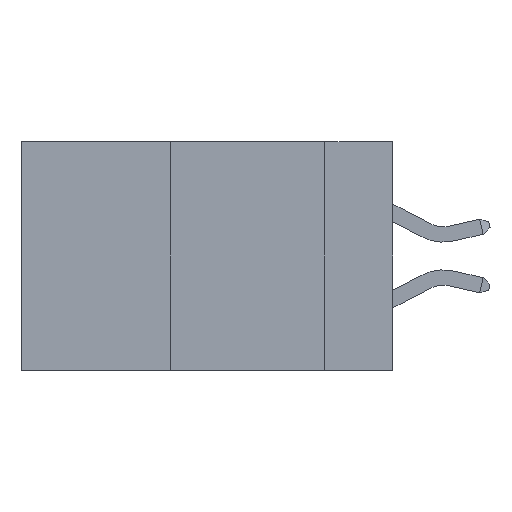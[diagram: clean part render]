
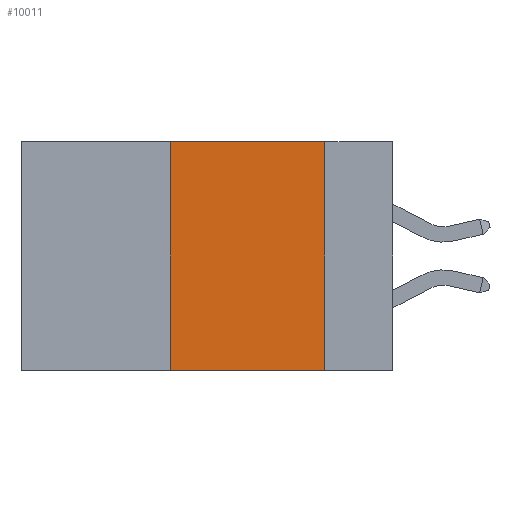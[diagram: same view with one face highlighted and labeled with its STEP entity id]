
A CAD part, left-side view. The second image highlights one B-rep face of the part: STEP entity #10011.
In plain terms, the highlighted planar face has unit normal (-1, 0, 0).
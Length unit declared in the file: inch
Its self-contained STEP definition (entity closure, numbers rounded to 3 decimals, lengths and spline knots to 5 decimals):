
#182 = VERTEX_POINT ( 'NONE', #9134 ) ;
#379 = VERTEX_POINT ( 'NONE', #16296 ) ;
#955 = EDGE_CURVE ( 'NONE', #4779, #379, #12647, .T. ) ;
#1255 = DIRECTION ( 'NONE',  ( 0., -1., 0. ) ) ;
#2209 = ORIENTED_EDGE ( 'NONE', *, *, #3180, .F. ) ;
#2214 = ORIENTED_EDGE ( 'NONE', *, *, #15296, .F. ) ;
#2442 = VECTOR ( 'NONE', #1255, 39.37008 ) ;
#2801 = CARTESIAN_POINT ( 'NONE',  ( 0., 0.36, -0.37 ) ) ;
#3041 = DIRECTION ( 'NONE',  ( 0., 0., -1. ) ) ;
#3180 = EDGE_CURVE ( 'NONE', #379, #4558, #3943, .T. ) ;
#3943 = LINE ( 'NONE', #12363, #13532 ) ;
#4366 = ORIENTED_EDGE ( 'NONE', *, *, #955, .F. ) ;
#4558 = VERTEX_POINT ( 'NONE', #12213 ) ;
#4779 = VERTEX_POINT ( 'NONE', #2801 ) ;
#5071 = AXIS2_PLACEMENT_3D ( 'NONE', #13150, #5720, #14394 ) ;
#5720 = DIRECTION ( 'NONE',  ( 1., 0., 0. ) ) ;
#8221 = PLANE ( 'NONE',  #5071 ) ;
#8478 = ORIENTED_EDGE ( 'NONE', *, *, #14471, .T. ) ;
#9134 = CARTESIAN_POINT ( 'NONE',  ( 0., 0.11, -0.37 ) ) ;
#9228 = DIRECTION ( 'NONE',  ( 0., 0., 1. ) ) ;
#9922 = DIRECTION ( 'NONE',  ( 0., -1., 0. ) ) ;
#10011 = ADVANCED_FACE ( 'NONE', ( #14382 ), #8221, .F. ) ;
#11688 = VECTOR ( 'NONE', #3041, 39.37008 ) ;
#12213 = CARTESIAN_POINT ( 'NONE',  ( 0., 0.11, 0. ) ) ;
#12254 = VECTOR ( 'NONE', #9228, 39.37008 ) ;
#12363 = CARTESIAN_POINT ( 'NONE',  ( 0., 0.6, 0. ) ) ;
#12644 = CARTESIAN_POINT ( 'NONE',  ( 0., 0.6, -0.37 ) ) ;
#12647 = LINE ( 'NONE', #14084, #12254 ) ;
#13150 = CARTESIAN_POINT ( 'NONE',  ( 0., 0.6, 0. ) ) ;
#13532 = VECTOR ( 'NONE', #9922, 39.37008 ) ;
#14084 = CARTESIAN_POINT ( 'NONE',  ( 0., 0.36, 0. ) ) ;
#14281 = CARTESIAN_POINT ( 'NONE',  ( 0., 0.11, 0. ) ) ;
#14382 = FACE_OUTER_BOUND ( 'NONE', #15607, .T. ) ;
#14394 = DIRECTION ( 'NONE',  ( 0., 0., -1. ) ) ;
#14471 = EDGE_CURVE ( 'NONE', #4779, #182, #15361, .T. ) ;
#14953 = LINE ( 'NONE', #14281, #11688 ) ;
#15296 = EDGE_CURVE ( 'NONE', #4558, #182, #14953, .T. ) ;
#15361 = LINE ( 'NONE', #12644, #2442 ) ;
#15607 = EDGE_LOOP ( 'NONE', ( #2214, #2209, #4366, #8478 ) ) ;
#16296 = CARTESIAN_POINT ( 'NONE',  ( 0., 0.36, 0. ) ) ;
